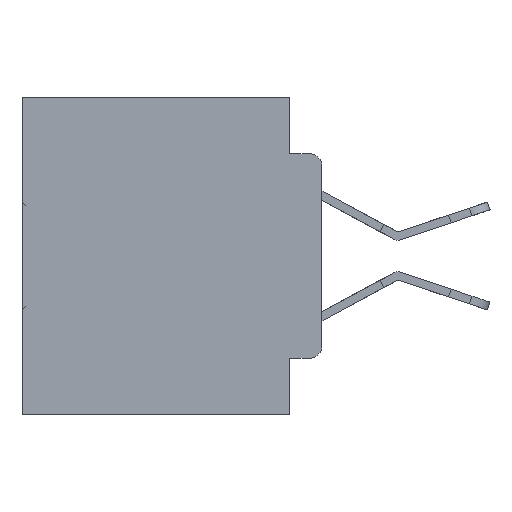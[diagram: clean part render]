
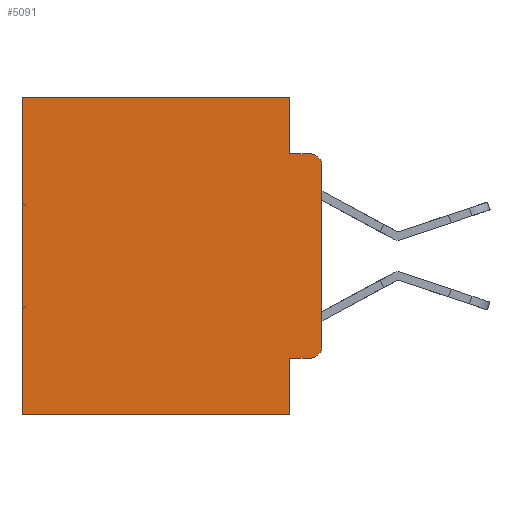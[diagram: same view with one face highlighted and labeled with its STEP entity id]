
A CAD part, left-side view. The second image highlights one B-rep face of the part: STEP entity #5091.
In plain terms, the highlighted planar face has unit normal (-1, 0, 0).
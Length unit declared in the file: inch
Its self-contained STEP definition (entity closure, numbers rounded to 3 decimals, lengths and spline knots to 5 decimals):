
#8 = CARTESIAN_POINT ( 'NONE',  ( 0.298, 0.02, -0.4115 ) ) ;
#637 = CARTESIAN_POINT ( 'NONE',  ( 0.298, 0., 0. ) ) ;
#784 = LINE ( 'NONE', #11938, #13560 ) ;
#902 = CARTESIAN_POINT ( 'NONE',  ( 0.298, 0.051, -0.0885 ) ) ;
#1284 = CIRCLE ( 'NONE', #23987, 0.02 ) ;
#2088 = ORIENTED_EDGE ( 'NONE', *, *, #32519, .F. ) ;
#2406 = VECTOR ( 'NONE', #4990, 39.37008 ) ;
#2575 = CARTESIAN_POINT ( 'NONE',  ( 0.298, 0.051, -0.4115 ) ) ;
#3582 = VERTEX_POINT ( 'NONE', #26038 ) ;
#3705 = CARTESIAN_POINT ( 'NONE',  ( 0.298, 0., -0.5 ) ) ;
#4343 = VERTEX_POINT ( 'NONE', #902 ) ;
#4762 = DIRECTION ( 'NONE',  ( 0., 1., 0. ) ) ;
#4990 = DIRECTION ( 'NONE',  ( 0., -1., 0. ) ) ;
#5091 = ADVANCED_FACE ( 'NONE', ( #24388 ), #33519, .F. ) ;
#5743 = VERTEX_POINT ( 'NONE', #29042 ) ;
#6176 = VECTOR ( 'NONE', #35988, 39.37008 ) ;
#6378 = ORIENTED_EDGE ( 'NONE', *, *, #11815, .F. ) ;
#7737 = CARTESIAN_POINT ( 'NONE',  ( 0.298, 0.051, -0.4115 ) ) ;
#8046 = VERTEX_POINT ( 'NONE', #23403 ) ;
#8336 = VECTOR ( 'NONE', #15169, 39.37008 ) ;
#8383 = VERTEX_POINT ( 'NONE', #8 ) ;
#8665 = EDGE_CURVE ( 'NONE', #12632, #23553, #29567, .T. ) ;
#8681 = LINE ( 'NONE', #637, #19135 ) ;
#9657 = DIRECTION ( 'NONE',  ( 0., 0., -1. ) ) ;
#11815 = EDGE_CURVE ( 'NONE', #17488, #26704, #33060, .T. ) ;
#11838 = ORIENTED_EDGE ( 'NONE', *, *, #28912, .T. ) ;
#11938 = CARTESIAN_POINT ( 'NONE',  ( 0.298, 0.051, -0.0885 ) ) ;
#12632 = VERTEX_POINT ( 'NONE', #25851 ) ;
#13560 = VECTOR ( 'NONE', #26866, 39.37008 ) ;
#13802 = ORIENTED_EDGE ( 'NONE', *, *, #30393, .F. ) ;
#13995 = CARTESIAN_POINT ( 'NONE',  ( 0.298, 0., 0. ) ) ;
#14335 = DIRECTION ( 'NONE',  ( 0., 0., -1. ) ) ;
#14659 = LINE ( 'NONE', #3705, #21421 ) ;
#15133 = EDGE_CURVE ( 'NONE', #3582, #8046, #23838, .T. ) ;
#15169 = DIRECTION ( 'NONE',  ( 0., 0., -1. ) ) ;
#15329 = EDGE_CURVE ( 'NONE', #3582, #5743, #8681, .T. ) ;
#15984 = CARTESIAN_POINT ( 'NONE',  ( 0.298, 0.473, -0.5 ) ) ;
#16726 = DIRECTION ( 'NONE',  ( 0., 0., -1. ) ) ;
#16920 = DIRECTION ( 'NONE',  ( 1., 0., 0. ) ) ;
#17178 = CARTESIAN_POINT ( 'NONE',  ( 0.298, 0.051, 0. ) ) ;
#17488 = VERTEX_POINT ( 'NONE', #2575 ) ;
#19135 = VECTOR ( 'NONE', #14335, 39.37008 ) ;
#19170 = ORIENTED_EDGE ( 'NONE', *, *, #8665, .T. ) ;
#19716 = EDGE_CURVE ( 'NONE', #20518, #12632, #29791, .T. ) ;
#20201 = ORIENTED_EDGE ( 'NONE', *, *, #15329, .F. ) ;
#20518 = VERTEX_POINT ( 'NONE', #27801 ) ;
#20702 = ORIENTED_EDGE ( 'NONE', *, *, #31006, .T. ) ;
#21421 = VECTOR ( 'NONE', #23046, 39.37008 ) ;
#22076 = DIRECTION ( 'NONE',  ( 0., 0., -1. ) ) ;
#23046 = DIRECTION ( 'NONE',  ( 0., 1., 0. ) ) ;
#23403 = CARTESIAN_POINT ( 'NONE',  ( 0.298, 0.02, -0.0885 ) ) ;
#23553 = VERTEX_POINT ( 'NONE', #15984 ) ;
#23838 = CIRCLE ( 'NONE', #30220, 0.02 ) ;
#23987 = AXIS2_PLACEMENT_3D ( 'NONE', #33221, #24788, #22076 ) ;
#24388 = FACE_OUTER_BOUND ( 'NONE', #30421, .T. ) ;
#24788 = DIRECTION ( 'NONE',  ( -1., 0., 0. ) ) ;
#25745 = ORIENTED_EDGE ( 'NONE', *, *, #19716, .T. ) ;
#25851 = CARTESIAN_POINT ( 'NONE',  ( 0.298, 0.473, 0. ) ) ;
#26038 = CARTESIAN_POINT ( 'NONE',  ( 0.298, 0., -0.1085 ) ) ;
#26262 = CARTESIAN_POINT ( 'NONE',  ( 0.298, 0.02, -0.1085 ) ) ;
#26704 = VERTEX_POINT ( 'NONE', #35513 ) ;
#26827 = EDGE_CURVE ( 'NONE', #26704, #23553, #14659, .T. ) ;
#26866 = DIRECTION ( 'NONE',  ( 0., -1., 0. ) ) ;
#27274 = VECTOR ( 'NONE', #4762, 39.37008 ) ;
#27801 = CARTESIAN_POINT ( 'NONE',  ( 0.298, 0.051, 0. ) ) ;
#28912 = EDGE_CURVE ( 'NONE', #17488, #8383, #32761, .T. ) ;
#29042 = CARTESIAN_POINT ( 'NONE',  ( 0.298, 0., -0.3915 ) ) ;
#29166 = ORIENTED_EDGE ( 'NONE', *, *, #26827, .F. ) ;
#29567 = LINE ( 'NONE', #32676, #32770 ) ;
#29791 = LINE ( 'NONE', #35459, #27274 ) ;
#30220 = AXIS2_PLACEMENT_3D ( 'NONE', #26262, #31759, #32130 ) ;
#30393 = EDGE_CURVE ( 'NONE', #4343, #8046, #784, .T. ) ;
#30421 = EDGE_LOOP ( 'NONE', ( #20201, #31541, #13802, #2088, #25745, #19170, #29166, #6378, #11838, #20702 ) ) ;
#31006 = EDGE_CURVE ( 'NONE', #8383, #5743, #1284, .T. ) ;
#31541 = ORIENTED_EDGE ( 'NONE', *, *, #15133, .T. ) ;
#31605 = LINE ( 'NONE', #17178, #8336 ) ;
#31759 = DIRECTION ( 'NONE',  ( -1., 0., 0. ) ) ;
#32043 = CARTESIAN_POINT ( 'NONE',  ( 0.298, 0.051, 0. ) ) ;
#32130 = DIRECTION ( 'NONE',  ( 0., 0., -1. ) ) ;
#32519 = EDGE_CURVE ( 'NONE', #20518, #4343, #31605, .T. ) ;
#32676 = CARTESIAN_POINT ( 'NONE',  ( 0.298, 0.473, 0. ) ) ;
#32761 = LINE ( 'NONE', #7737, #2406 ) ;
#32770 = VECTOR ( 'NONE', #9657, 39.37008 ) ;
#33060 = LINE ( 'NONE', #32043, #6176 ) ;
#33221 = CARTESIAN_POINT ( 'NONE',  ( 0.298, 0.02, -0.3915 ) ) ;
#33519 = PLANE ( 'NONE',  #33842 ) ;
#33842 = AXIS2_PLACEMENT_3D ( 'NONE', #13995, #16920, #16726 ) ;
#35459 = CARTESIAN_POINT ( 'NONE',  ( 0.298, 0., 0. ) ) ;
#35513 = CARTESIAN_POINT ( 'NONE',  ( 0.298, 0.051, -0.5 ) ) ;
#35988 = DIRECTION ( 'NONE',  ( 0., 0., -1. ) ) ;
